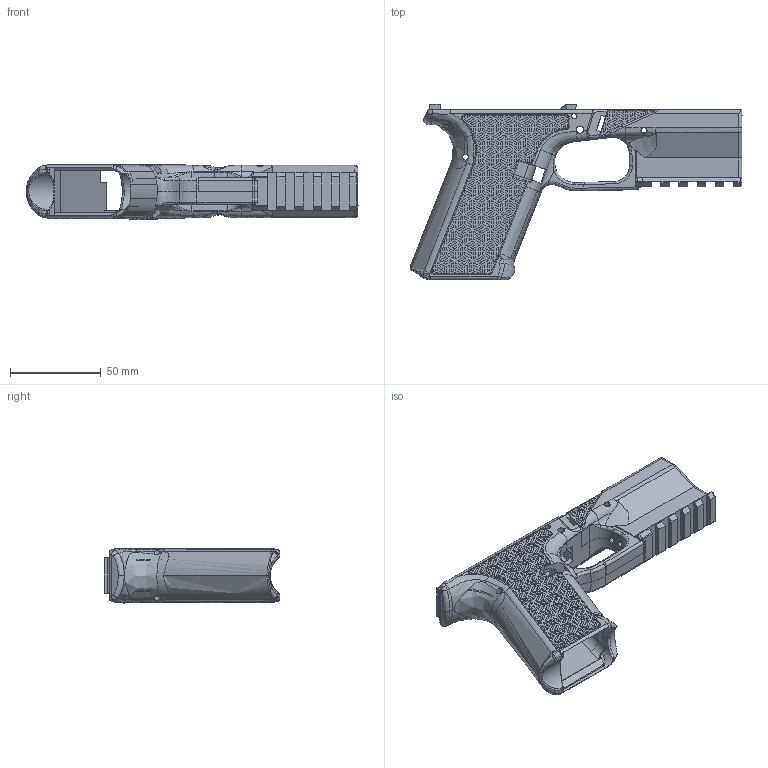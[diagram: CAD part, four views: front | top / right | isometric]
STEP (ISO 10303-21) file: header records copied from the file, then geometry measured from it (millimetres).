
FILE_DESCRIPTION(/* description */ (''),/* implementation_level */ '2;1');
FILE_NAME(/* name */ 'Lil Chungus Full Stipple.step',/* time_stamp */ '2021-04-29T09:19:44-06:00',/* author */ (''),/* organization */ (''),/* preprocessor_version */ 'ST-DEVELOPER v18.1',/* originating_system */ 'Autodesk Translation Framework v10.6.0.1341',/* authorisation */ '');
FILE_SCHEMA (('AUTOMOTIVE_DESIGN { 1 0 10303 214 3 1 1 }'));
Products named in the file (1): Lil Chungus Big Grips
Bounding box: 183.22 x 97 x 30.34 mm (x, y, z)
Volume: 102940.7 mm3; surface area: 54353.6 mm2
Topology: 1 solids, 6 shells, 5241 faces, 14100 edges, 9197 vertices
Faces by surface type: plane 2797, bspline 2139, cylinder 236, torus 50, sphere 16, cone 3
Full cylindrical faces by diameter (mm): 2 x1, 3 x4, 3.2 x2, 4 x2
Entity records: 192434 total; most frequent: CARTESIAN_POINT 81188, ORIENTED_EDGE 28184, DIRECTION 16749, EDGE_CURVE 14092, VERTEX_POINT 9198, LINE 8961, VECTOR 8961, EDGE_LOOP 5612
